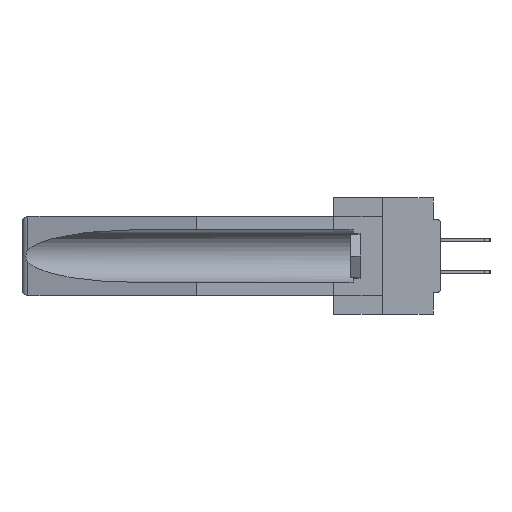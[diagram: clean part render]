
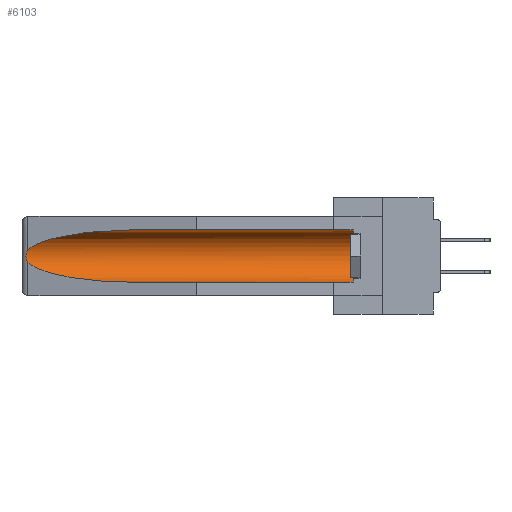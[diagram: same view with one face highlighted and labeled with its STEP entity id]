
A CAD part, left-side view. The second image highlights one B-rep face of the part: STEP entity #6103.
In plain terms, the highlighted cylindrical face has radius 2.857 mm (diameter 5.715 mm), a partial arc.
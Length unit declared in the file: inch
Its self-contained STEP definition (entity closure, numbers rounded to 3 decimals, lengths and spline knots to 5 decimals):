
#594 = ORIENTED_EDGE ( 'NONE', *, *, #5438, .T. ) ;
#1144 = VERTEX_POINT ( 'NONE', #10735 ) ;
#1565 = EDGE_CURVE ( 'NONE', #22525, #38275, #19566, .T. ) ;
#1672 = CARTESIAN_POINT ( 'NONE',  ( 0.26537, 1.52718, -0.19328 ) ) ;
#1742 = CARTESIAN_POINT ( 'NONE',  ( 0.155, 1.07973, -0.284 ) ) ;
#1787 = CYLINDRICAL_SURFACE ( 'NONE', #26980, 0.1125 ) ;
#4971 = VERTEX_POINT ( 'NONE', #40439 ) ;
#5004 = CARTESIAN_POINT ( 'NONE',  ( 0.26597, 1.5296, -0.19026 ) ) ;
#5438 = EDGE_CURVE ( 'NONE', #1144, #23280, #34354, .T. ) ;
#5917 = DIRECTION ( 'NONE',  ( 0., 1., 0. ) ) ;
#6103 = ADVANCED_FACE ( 'NONE', ( #6273 ), #1787, .F. ) ;
#6122 = CARTESIAN_POINT ( 'NONE',  ( 0.155, -0.30754, -0.059 ) ) ;
#6130 = CARTESIAN_POINT ( 'NONE',  ( 0.26537, 1.52718, -0.14972 ) ) ;
#6273 = FACE_OUTER_BOUND ( 'NONE', #34483, .T. ) ;
#6454 = EDGE_CURVE ( 'NONE', #23280, #41061, #15835, .T. ) ;
#7296 = CARTESIAN_POINT ( 'NONE',  ( 0.155, 0.126, -0.284 ) ) ;
#7988 = CARTESIAN_POINT ( 'NONE',  ( 0.155, 0.126, -0.1715 ) ) ;
#8762 = CARTESIAN_POINT ( 'NONE',  ( 0.21114, 1.30732, -0.059 ) ) ;
#10735 = CARTESIAN_POINT ( 'NONE',  ( 0.155, 1.07973, -0.059 ) ) ;
#10775 = CARTESIAN_POINT ( 'NONE',  ( 0.155, -0.30754, -0.284 ) ) ;
#11168 = EDGE_CURVE ( 'NONE', #41061, #38275, #33602, .T. ) ;
#11637 = CARTESIAN_POINT ( 'NONE',  ( 0.155, -0.30754, -0.1715 ) ) ;
#12148 = ORIENTED_EDGE ( 'NONE', *, *, #1565, .F. ) ;
#12505 = CARTESIAN_POINT ( 'NONE',  ( 0.26537, 1.52718, -0.14972 ) ) ;
#13232 = CARTESIAN_POINT ( 'NONE',  ( 0.26537, 1.52718, -0.19328 ) ) ;
#13565 = VECTOR ( 'NONE', #36123, 39.37008 ) ;
#14312 = CARTESIAN_POINT ( 'NONE',  ( 0.2675, 1.53308, -0.17534 ) ) ;
#14714 = ORIENTED_EDGE ( 'NONE', *, *, #28626, .T. ) ;
#15835 = B_SPLINE_CURVE_WITH_KNOTS ( 'NONE', 3,
 ( #26829, #17649, #39522, #32896, #23795, #14312, #36459, #17511, #5004, #1672 ),
 .UNSPECIFIED., .F., .F.,
 ( 4, 2, 2, 2, 4 ),
 ( 0., 0.00029, 0.00058, 0.00087, 0.00117 ),
 .UNSPECIFIED. ) ;
#17511 = CARTESIAN_POINT ( 'NONE',  ( 0.26655, 1.53094, -0.18657 ) ) ;
#17649 = CARTESIAN_POINT ( 'NONE',  ( 0.26597, 1.52961, -0.15275 ) ) ;
#17829 = VECTOR ( 'NONE', #21713, 39.37008 ) ;
#18825 = CARTESIAN_POINT ( 'NONE',  ( 0.25451, 1.48313, -0.24835 ) ) ;
#19523 = EDGE_CURVE ( 'NONE', #4971, #1144, #35141, .T. ) ;
#19566 = LINE ( 'NONE', #10775, #13565 ) ;
#21555 = CARTESIAN_POINT ( 'NONE',  ( 0.25451, 1.48313, -0.09465 ) ) ;
#21697 = CARTESIAN_POINT ( 'NONE',  ( 0.155, 1.07973, -0.059 ) ) ;
#21713 = DIRECTION ( 'NONE',  ( 0., 1., 0. ) ) ;
#22525 = VERTEX_POINT ( 'NONE', #7296 ) ;
#23280 = VERTEX_POINT ( 'NONE', #6130 ) ;
#23795 = CARTESIAN_POINT ( 'NONE',  ( 0.2675, 1.53308, -0.16763 ) ) ;
#26829 = CARTESIAN_POINT ( 'NONE',  ( 0.26537, 1.52718, -0.14972 ) ) ;
#26980 = AXIS2_PLACEMENT_3D ( 'NONE', #11637, #5917, #34349 ) ;
#27150 = AXIS2_PLACEMENT_3D ( 'NONE', #7988, #33358, #30203 ) ;
#28626 = EDGE_CURVE ( 'NONE', #22525, #4971, #40548, .T. ) ;
#28667 = CARTESIAN_POINT ( 'NONE',  ( 0.155, 1.07973, -0.284 ) ) ;
#30203 = DIRECTION ( 'NONE',  ( 0., 0., 1. ) ) ;
#31586 = ORIENTED_EDGE ( 'NONE', *, *, #6454, .T. ) ;
#32896 = CARTESIAN_POINT ( 'NONE',  ( 0.2673, 1.5327, -0.16383 ) ) ;
#33358 = DIRECTION ( 'NONE',  ( 0., -1., 0. ) ) ;
#33602 =( BOUNDED_CURVE ( )  B_SPLINE_CURVE ( 3, ( #38164, #18825, #34721, #28667 ),
 .UNSPECIFIED., .F., .T. ) 
 B_SPLINE_CURVE_WITH_KNOTS ( ( 4, 4 ),
 ( 0.1948, 1.5708 ),
 .UNSPECIFIED. ) 
 CURVE ( )  GEOMETRIC_REPRESENTATION_ITEM ( )  RATIONAL_B_SPLINE_CURVE ( ( 1., 0.848, 0.848, 1. ) ) 
 REPRESENTATION_ITEM ( '' )  );
#34349 = DIRECTION ( 'NONE',  ( 0., 0., 1. ) ) ;
#34354 =( BOUNDED_CURVE ( )  B_SPLINE_CURVE ( 3, ( #21697, #8762, #21555, #12505 ),
 .UNSPECIFIED., .F., .F. ) 
 B_SPLINE_CURVE_WITH_KNOTS ( ( 4, 4 ),
 ( 4.71239, 6.08839 ),
 .UNSPECIFIED. ) 
 CURVE ( )  GEOMETRIC_REPRESENTATION_ITEM ( )  RATIONAL_B_SPLINE_CURVE ( ( 1., 0.848, 0.848, 1. ) ) 
 REPRESENTATION_ITEM ( '' )  );
#34483 = EDGE_LOOP ( 'NONE', ( #594, #31586, #36408, #12148, #14714, #40967 ) ) ;
#34721 = CARTESIAN_POINT ( 'NONE',  ( 0.21114, 1.30732, -0.284 ) ) ;
#35141 = LINE ( 'NONE', #6122, #17829 ) ;
#36123 = DIRECTION ( 'NONE',  ( 0., 1., 0. ) ) ;
#36408 = ORIENTED_EDGE ( 'NONE', *, *, #11168, .T. ) ;
#36459 = CARTESIAN_POINT ( 'NONE',  ( 0.2673, 1.53269, -0.17917 ) ) ;
#38164 = CARTESIAN_POINT ( 'NONE',  ( 0.26537, 1.52718, -0.19328 ) ) ;
#38275 = VERTEX_POINT ( 'NONE', #1742 ) ;
#39522 = CARTESIAN_POINT ( 'NONE',  ( 0.26654, 1.53092, -0.15636 ) ) ;
#40439 = CARTESIAN_POINT ( 'NONE',  ( 0.155, 0.126, -0.059 ) ) ;
#40548 = CIRCLE ( 'NONE', #27150, 0.1125 ) ;
#40967 = ORIENTED_EDGE ( 'NONE', *, *, #19523, .T. ) ;
#41061 = VERTEX_POINT ( 'NONE', #13232 ) ;
